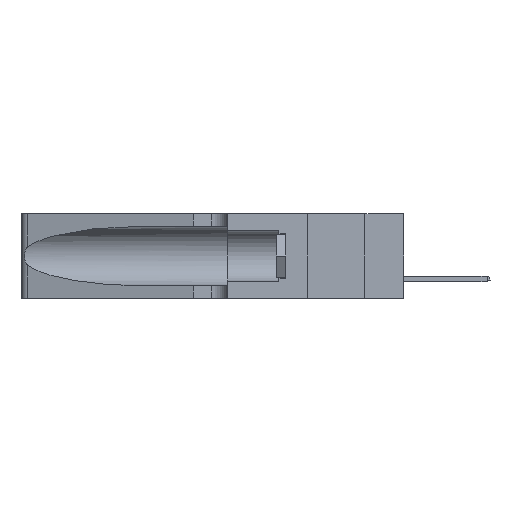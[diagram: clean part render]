
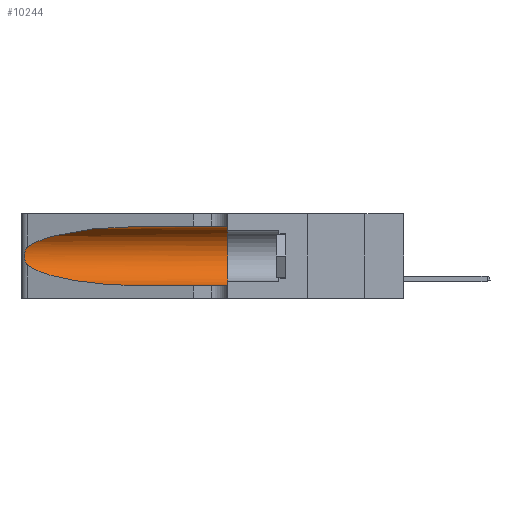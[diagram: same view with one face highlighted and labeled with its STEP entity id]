
A CAD part, left-side view. The second image highlights one B-rep face of the part: STEP entity #10244.
In plain terms, the highlighted cylindrical face has radius 3.308 mm (diameter 6.617 mm), a partial arc.
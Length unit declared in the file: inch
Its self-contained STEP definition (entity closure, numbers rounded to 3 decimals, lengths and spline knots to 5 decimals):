
#847 = CARTESIAN_POINT ( 'NONE',  ( 0.1305, 1.61858, 0.31525 ) ) ;
#1706 =( BOUNDED_CURVE ( )  B_SPLINE_CURVE ( 3, ( #2386, #4245, #2704, #17743 ),
 .UNSPECIFIED., .F., .T. ) 
 B_SPLINE_CURVE_WITH_KNOTS ( ( 4, 4 ),
 ( 1.5708, 2.84003 ),
 .UNSPECIFIED. ) 
 CURVE ( )  GEOMETRIC_REPRESENTATION_ITEM ( )  RATIONAL_B_SPLINE_CURVE ( ( 1., 0.87, 0.87, 1. ) ) 
 REPRESENTATION_ITEM ( '' )  );
#1798 = CARTESIAN_POINT ( 'NONE',  ( 0.25487, 1.22718, 0.22369 ) ) ;
#2000 = CARTESIAN_POINT ( 'NONE',  ( 0.25639, 1.23184, 0.21858 ) ) ;
#2386 = CARTESIAN_POINT ( 'NONE',  ( 0.1305, 0.72297, 0.31525 ) ) ;
#2431 = EDGE_CURVE ( 'NONE', #4103, #3742, #14727, .T. ) ;
#2610 = B_SPLINE_CURVE_WITH_KNOTS ( 'NONE', 3,
 ( #11374, #7636, #2000, #4267, #17176, #7791, #13675, #22815, #19112, #11800, #6028, #15574, #22735, #18864 ),
 .UNSPECIFIED., .F., .F.,
 ( 4, 2, 2, 2, 2, 2, 4 ),
 ( 0., 0.00027, 0.00053, 0.00107, 0.0016, 0.00187, 0.00214 ),
 .UNSPECIFIED. ) ;
#2704 = CARTESIAN_POINT ( 'NONE',  ( 0.2373, 1.15595, 0.28018 ) ) ;
#2909 = CARTESIAN_POINT ( 'NONE',  ( 0.25487, 1.22718, 0.14631 ) ) ;
#2943 = EDGE_CURVE ( 'NONE', #13722, #8535, #2610, .T. ) ;
#3671 = DIRECTION ( 'NONE',  ( 0., -1., 0. ) ) ;
#3742 = VERTEX_POINT ( 'NONE', #14198 ) ;
#4103 = VERTEX_POINT ( 'NONE', #7311 ) ;
#4245 = CARTESIAN_POINT ( 'NONE',  ( 0.18966, 0.96281, 0.31525 ) ) ;
#4267 = CARTESIAN_POINT ( 'NONE',  ( 0.25787, 1.23484, 0.2124 ) ) ;
#5247 = CARTESIAN_POINT ( 'NONE',  ( 0.1305, 0.72297, 0.31525 ) ) ;
#5488 = AXIS2_PLACEMENT_3D ( 'NONE', #16636, #22351, #16709 ) ;
#6028 = CARTESIAN_POINT ( 'NONE',  ( 0.25789, 1.23486, 0.15765 ) ) ;
#6376 = CYLINDRICAL_SURFACE ( 'NONE', #5488, 0.13025 ) ;
#6429 = VERTEX_POINT ( 'NONE', #5247 ) ;
#6846 = VECTOR ( 'NONE', #3671, 39.37008 ) ;
#7311 = CARTESIAN_POINT ( 'NONE',  ( 0.1305, 0.72297, 0.05475 ) ) ;
#7636 = CARTESIAN_POINT ( 'NONE',  ( 0.25555, 1.22994, 0.2215 ) ) ;
#7791 = CARTESIAN_POINT ( 'NONE',  ( 0.26018, 1.23835, 0.19895 ) ) ;
#7897 = EDGE_CURVE ( 'NONE', #13507, #3742, #21105, .T. ) ;
#8255 = ORIENTED_EDGE ( 'NONE', *, *, #19322, .T. ) ;
#8535 = VERTEX_POINT ( 'NONE', #13350 ) ;
#9045 = ORIENTED_EDGE ( 'NONE', *, *, #2431, .T. ) ;
#10244 = ADVANCED_FACE ( 'NONE', ( #12482 ), #6376, .F. ) ;
#10342 =( BOUNDED_CURVE ( )  B_SPLINE_CURVE ( 3, ( #2909, #15999, #12540, #18782 ),
 .UNSPECIFIED., .F., .T. ) 
 B_SPLINE_CURVE_WITH_KNOTS ( ( 4, 4 ),
 ( 3.44316, 4.71239 ),
 .UNSPECIFIED. ) 
 CURVE ( )  GEOMETRIC_REPRESENTATION_ITEM ( )  RATIONAL_B_SPLINE_CURVE ( ( 1., 0.87, 0.87, 1. ) ) 
 REPRESENTATION_ITEM ( '' )  );
#11374 = CARTESIAN_POINT ( 'NONE',  ( 0.25487, 1.22718, 0.22369 ) ) ;
#11783 = EDGE_LOOP ( 'NONE', ( #8255, #22371, #20808, #9045, #19334, #16486 ) ) ;
#11800 = CARTESIAN_POINT ( 'NONE',  ( 0.25856, 1.23593, 0.16098 ) ) ;
#12482 = FACE_OUTER_BOUND ( 'NONE', #11783, .T. ) ;
#12540 = CARTESIAN_POINT ( 'NONE',  ( 0.18966, 0.96281, 0.05475 ) ) ;
#12742 = DIRECTION ( 'NONE',  ( 0., -1., 0. ) ) ;
#12904 = LINE ( 'NONE', #847, #17619 ) ;
#12956 = EDGE_CURVE ( 'NONE', #6429, #13507, #12904, .T. ) ;
#13350 = CARTESIAN_POINT ( 'NONE',  ( 0.25487, 1.22718, 0.14631 ) ) ;
#13507 = VERTEX_POINT ( 'NONE', #14540 ) ;
#13675 = CARTESIAN_POINT ( 'NONE',  ( 0.26075, 1.23896, 0.19203 ) ) ;
#13722 = VERTEX_POINT ( 'NONE', #1798 ) ;
#14198 = CARTESIAN_POINT ( 'NONE',  ( 0.1305, 0.35, 0.05475 ) ) ;
#14540 = CARTESIAN_POINT ( 'NONE',  ( 0.1305, 0.35, 0.31525 ) ) ;
#14727 = LINE ( 'NONE', #14802, #6846 ) ;
#14802 = CARTESIAN_POINT ( 'NONE',  ( 0.1305, 1.61858, 0.05475 ) ) ;
#15574 = CARTESIAN_POINT ( 'NONE',  ( 0.25639, 1.23186, 0.15144 ) ) ;
#15981 = EDGE_CURVE ( 'NONE', #8535, #4103, #10342, .T. ) ;
#15999 = CARTESIAN_POINT ( 'NONE',  ( 0.2373, 1.15595, 0.08982 ) ) ;
#16133 = CARTESIAN_POINT ( 'NONE',  ( 0.1305, 0.35, 0.185 ) ) ;
#16486 = ORIENTED_EDGE ( 'NONE', *, *, #12956, .F. ) ;
#16636 = CARTESIAN_POINT ( 'NONE',  ( 0.1305, 1.61858, 0.185 ) ) ;
#16709 = DIRECTION ( 'NONE',  ( 0., 0., -1. ) ) ;
#17176 = CARTESIAN_POINT ( 'NONE',  ( 0.25854, 1.2359, 0.20912 ) ) ;
#17619 = VECTOR ( 'NONE', #12742, 39.37008 ) ;
#17743 = CARTESIAN_POINT ( 'NONE',  ( 0.25487, 1.22718, 0.22369 ) ) ;
#18782 = CARTESIAN_POINT ( 'NONE',  ( 0.1305, 0.72297, 0.05475 ) ) ;
#18864 = CARTESIAN_POINT ( 'NONE',  ( 0.25487, 1.22718, 0.14631 ) ) ;
#19112 = CARTESIAN_POINT ( 'NONE',  ( 0.26017, 1.23833, 0.17102 ) ) ;
#19322 = EDGE_CURVE ( 'NONE', #6429, #13722, #1706, .T. ) ;
#19334 = ORIENTED_EDGE ( 'NONE', *, *, #7897, .F. ) ;
#19821 = DIRECTION ( 'NONE',  ( 0., 1., 0. ) ) ;
#19893 = DIRECTION ( 'NONE',  ( 0., 0., 1. ) ) ;
#20808 = ORIENTED_EDGE ( 'NONE', *, *, #15981, .T. ) ;
#21105 = CIRCLE ( 'NONE', #22382, 0.13025 ) ;
#22351 = DIRECTION ( 'NONE',  ( 0., -1., 0. ) ) ;
#22371 = ORIENTED_EDGE ( 'NONE', *, *, #2943, .T. ) ;
#22382 = AXIS2_PLACEMENT_3D ( 'NONE', #16133, #19821, #19893 ) ;
#22735 = CARTESIAN_POINT ( 'NONE',  ( 0.25555, 1.22993, 0.14849 ) ) ;
#22815 = CARTESIAN_POINT ( 'NONE',  ( 0.26075, 1.23896, 0.178 ) ) ;
